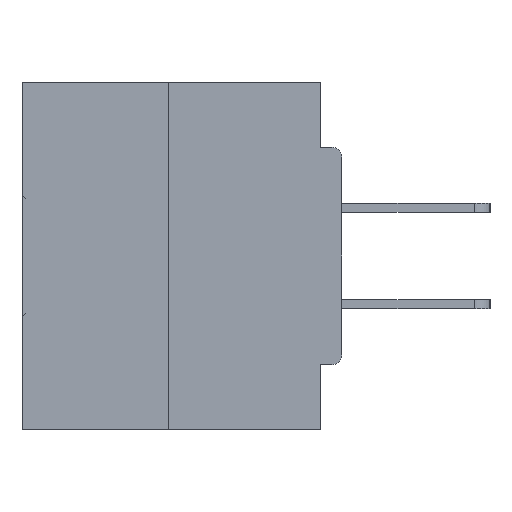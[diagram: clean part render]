
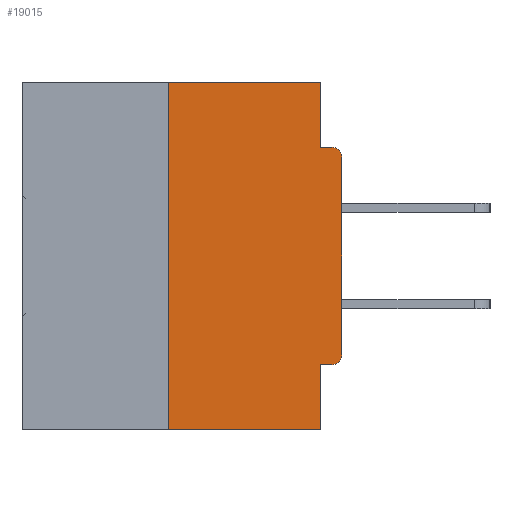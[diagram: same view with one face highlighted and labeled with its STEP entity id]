
A CAD part, left-side view. The second image highlights one B-rep face of the part: STEP entity #19015.
In plain terms, the highlighted planar face has unit normal (-1, 0, 0).
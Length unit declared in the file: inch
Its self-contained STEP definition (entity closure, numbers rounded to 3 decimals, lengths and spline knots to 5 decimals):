
#210 = ORIENTED_EDGE ( 'NONE', *, *, #1353, .T. ) ;
#826 = LINE ( 'NONE', #3473, #28178 ) ;
#1161 = CARTESIAN_POINT ( 'NONE',  ( 0., 0.031, 0. ) ) ;
#1353 = EDGE_CURVE ( 'NONE', #18352, #30442, #6815, .T. ) ;
#2901 = CARTESIAN_POINT ( 'NONE',  ( 0., 0.25, -0.5 ) ) ;
#3129 = VECTOR ( 'NONE', #16929, 39.37008 ) ;
#3473 = CARTESIAN_POINT ( 'NONE',  ( 0., 0.031, -0.5 ) ) ;
#3525 = EDGE_CURVE ( 'NONE', #16158, #30442, #24912, .T. ) ;
#5902 = EDGE_CURVE ( 'NONE', #27471, #16158, #35515, .T. ) ;
#6353 = VERTEX_POINT ( 'NONE', #27967 ) ;
#6815 = CIRCLE ( 'NONE', #20641, 0.015 ) ;
#7101 = EDGE_LOOP ( 'NONE', ( #13213, #10915, #17192, #18382, #43418, #28102, #12209, #210, #12634, #44419 ) ) ;
#8403 = DIRECTION ( 'NONE',  ( 0., -1., 0. ) ) ;
#8933 = EDGE_CURVE ( 'NONE', #6353, #27471, #20691, .T. ) ;
#9251 = VECTOR ( 'NONE', #20092, 39.37008 ) ;
#9920 = CARTESIAN_POINT ( 'NONE',  ( 0., 0., -0.0935 ) ) ;
#10039 = DIRECTION ( 'NONE',  ( 0., 0., -1. ) ) ;
#10589 = PLANE ( 'NONE',  #13292 ) ;
#10643 = FACE_OUTER_BOUND ( 'NONE', #7101, .T. ) ;
#10915 = ORIENTED_EDGE ( 'NONE', *, *, #29565, .F. ) ;
#12209 = ORIENTED_EDGE ( 'NONE', *, *, #38264, .T. ) ;
#12559 = CIRCLE ( 'NONE', #16714, 0.015 ) ;
#12634 = ORIENTED_EDGE ( 'NONE', *, *, #3525, .F. ) ;
#13003 = CARTESIAN_POINT ( 'NONE',  ( 0., 0.015, -0.1085 ) ) ;
#13213 = ORIENTED_EDGE ( 'NONE', *, *, #8933, .F. ) ;
#13292 = AXIS2_PLACEMENT_3D ( 'NONE', #34640, #20930, #42737 ) ;
#14069 = CARTESIAN_POINT ( 'NONE',  ( 0., 0., 0. ) ) ;
#14126 = DIRECTION ( 'NONE',  ( 0., 0., -1. ) ) ;
#14428 = VERTEX_POINT ( 'NONE', #38011 ) ;
#14955 = LINE ( 'NONE', #28888, #25698 ) ;
#16009 = VERTEX_POINT ( 'NONE', #21049 ) ;
#16158 = VERTEX_POINT ( 'NONE', #22397 ) ;
#16714 = AXIS2_PLACEMENT_3D ( 'NONE', #43364, #19050, #29484 ) ;
#16929 = DIRECTION ( 'NONE',  ( 0., 0., 1. ) ) ;
#17192 = ORIENTED_EDGE ( 'NONE', *, *, #29439, .T. ) ;
#18352 = VERTEX_POINT ( 'NONE', #35794 ) ;
#18382 = ORIENTED_EDGE ( 'NONE', *, *, #33120, .F. ) ;
#19015 = ADVANCED_FACE ( 'NONE', ( #10643 ), #10589, .F. ) ;
#19050 = DIRECTION ( 'NONE',  ( -1., 0., 0. ) ) ;
#19201 = DIRECTION ( 'NONE',  ( 0., -1., 0. ) ) ;
#19954 = VECTOR ( 'NONE', #19201, 39.37008 ) ;
#20092 = DIRECTION ( 'NONE',  ( 0., 0., 1. ) ) ;
#20247 = CARTESIAN_POINT ( 'NONE',  ( 0., 0.031, 0. ) ) ;
#20641 = AXIS2_PLACEMENT_3D ( 'NONE', #13003, #23361, #36490 ) ;
#20691 = LINE ( 'NONE', #39270, #35799 ) ;
#20930 = DIRECTION ( 'NONE',  ( 1., 0., 0. ) ) ;
#21030 = LINE ( 'NONE', #39884, #19954 ) ;
#21049 = CARTESIAN_POINT ( 'NONE',  ( 0., 0.031, -0.5 ) ) ;
#21376 = LINE ( 'NONE', #14069, #3129 ) ;
#22397 = CARTESIAN_POINT ( 'NONE',  ( 0., 0.031, -0.0935 ) ) ;
#22969 = CARTESIAN_POINT ( 'NONE',  ( 0., 0., -0.3915 ) ) ;
#23361 = DIRECTION ( 'NONE',  ( -1., 0., 0. ) ) ;
#23747 = EDGE_CURVE ( 'NONE', #31556, #14428, #14955, .T. ) ;
#24912 = LINE ( 'NONE', #9920, #34092 ) ;
#25698 = VECTOR ( 'NONE', #39015, 39.37008 ) ;
#26360 = VECTOR ( 'NONE', #10039, 39.37008 ) ;
#27471 = VERTEX_POINT ( 'NONE', #1161 ) ;
#27967 = CARTESIAN_POINT ( 'NONE',  ( 0., 0.25, 0. ) ) ;
#28102 = ORIENTED_EDGE ( 'NONE', *, *, #28542, .T. ) ;
#28178 = VECTOR ( 'NONE', #14126, 39.37008 ) ;
#28542 = EDGE_CURVE ( 'NONE', #31556, #30728, #12559, .T. ) ;
#28888 = CARTESIAN_POINT ( 'NONE',  ( 0., 0., -0.4065 ) ) ;
#29439 = EDGE_CURVE ( 'NONE', #37679, #16009, #21030, .T. ) ;
#29484 = DIRECTION ( 'NONE',  ( 0., 0., -1. ) ) ;
#29565 = EDGE_CURVE ( 'NONE', #37679, #6353, #44278, .T. ) ;
#30442 = VERTEX_POINT ( 'NONE', #32033 ) ;
#30728 = VERTEX_POINT ( 'NONE', #22969 ) ;
#31556 = VERTEX_POINT ( 'NONE', #35934 ) ;
#32033 = CARTESIAN_POINT ( 'NONE',  ( 0., 0.015, -0.0935 ) ) ;
#33120 = EDGE_CURVE ( 'NONE', #14428, #16009, #826, .T. ) ;
#33811 = CARTESIAN_POINT ( 'NONE',  ( 0., 0.25, 0. ) ) ;
#34092 = VECTOR ( 'NONE', #37203, 39.37008 ) ;
#34640 = CARTESIAN_POINT ( 'NONE',  ( 0., 0.46, 0. ) ) ;
#35515 = LINE ( 'NONE', #20247, #26360 ) ;
#35794 = CARTESIAN_POINT ( 'NONE',  ( 0., 0., -0.1085 ) ) ;
#35799 = VECTOR ( 'NONE', #8403, 39.37008 ) ;
#35934 = CARTESIAN_POINT ( 'NONE',  ( 0., 0.015, -0.4065 ) ) ;
#36490 = DIRECTION ( 'NONE',  ( 0., 0., -1. ) ) ;
#37203 = DIRECTION ( 'NONE',  ( 0., -1., 0. ) ) ;
#37679 = VERTEX_POINT ( 'NONE', #2901 ) ;
#38011 = CARTESIAN_POINT ( 'NONE',  ( 0., 0.031, -0.4065 ) ) ;
#38264 = EDGE_CURVE ( 'NONE', #30728, #18352, #21376, .T. ) ;
#39015 = DIRECTION ( 'NONE',  ( 0., 1., 0. ) ) ;
#39270 = CARTESIAN_POINT ( 'NONE',  ( 0., 0.46, 0. ) ) ;
#39884 = CARTESIAN_POINT ( 'NONE',  ( 0., 0.46, -0.5 ) ) ;
#42737 = DIRECTION ( 'NONE',  ( 0., 0., -1. ) ) ;
#43364 = CARTESIAN_POINT ( 'NONE',  ( 0., 0.015, -0.3915 ) ) ;
#43418 = ORIENTED_EDGE ( 'NONE', *, *, #23747, .F. ) ;
#44278 = LINE ( 'NONE', #33811, #9251 ) ;
#44419 = ORIENTED_EDGE ( 'NONE', *, *, #5902, .F. ) ;
